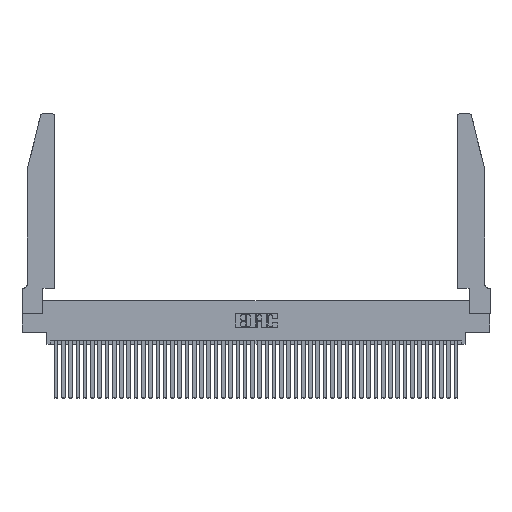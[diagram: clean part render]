
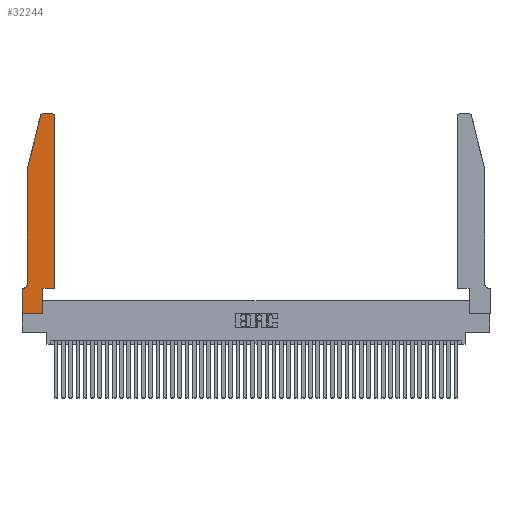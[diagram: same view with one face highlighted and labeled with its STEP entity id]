
A CAD part, top view. The second image highlights one B-rep face of the part: STEP entity #32244.
In plain terms, the highlighted planar face has unit normal (0, 0, 1).
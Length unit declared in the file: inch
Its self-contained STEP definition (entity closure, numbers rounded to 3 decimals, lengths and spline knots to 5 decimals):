
#1064 = EDGE_CURVE ( 'NONE', #2096, #32470, #44818, .T. ) ;
#1934 = DIRECTION ( 'NONE',  ( 0., -1., 0. ) ) ;
#2096 = VERTEX_POINT ( 'NONE', #42912 ) ;
#3128 = ORIENTED_EDGE ( 'NONE', *, *, #29741, .T. ) ;
#4779 = VECTOR ( 'NONE', #26442, 39.37008 ) ;
#6414 = LINE ( 'NONE', #42058, #39681 ) ;
#6590 = VECTOR ( 'NONE', #1934, 39.37008 ) ;
#6786 = CARTESIAN_POINT ( 'NONE',  ( 0.4505, 2.72, 0.37 ) ) ;
#6930 = VECTOR ( 'NONE', #35611, 39.37008 ) ;
#6940 = EDGE_CURVE ( 'NONE', #19842, #30577, #6414, .T. ) ;
#7365 = DIRECTION ( 'NONE',  ( 1., 0., 0. ) ) ;
#8412 = ORIENTED_EDGE ( 'NONE', *, *, #44773, .T. ) ;
#9983 = LINE ( 'NONE', #26506, #6590 ) ;
#10655 = PLANE ( 'NONE',  #27643 ) ;
#12124 = CARTESIAN_POINT ( 'NONE',  ( 0.0755, 0.35, 0.37 ) ) ;
#12376 = CARTESIAN_POINT ( 'NONE',  ( 0.2865, 0.35, 0.37 ) ) ;
#12645 = CARTESIAN_POINT ( 'NONE',  ( 0., 0.35, 0.37 ) ) ;
#13180 = VERTEX_POINT ( 'NONE', #37721 ) ;
#14116 = FACE_OUTER_BOUND ( 'NONE', #36473, .T. ) ;
#14695 = ORIENTED_EDGE ( 'NONE', *, *, #1064, .T. ) ;
#14937 = VECTOR ( 'NONE', #29112, 39.37008 ) ;
#15252 = VERTEX_POINT ( 'NONE', #18741 ) ;
#15470 = LINE ( 'NONE', #26940, #4779 ) ;
#15561 = VECTOR ( 'NONE', #19026, 39.37008 ) ;
#15694 = DIRECTION ( 'NONE',  ( 0., 1., 0. ) ) ;
#15696 = VERTEX_POINT ( 'NONE', #40774 ) ;
#15975 = ORIENTED_EDGE ( 'NONE', *, *, #6940, .T. ) ;
#17004 = ORIENTED_EDGE ( 'NONE', *, *, #36597, .T. ) ;
#17228 = VERTEX_POINT ( 'NONE', #45197 ) ;
#17938 = CARTESIAN_POINT ( 'NONE',  ( 0.4505, 0.35, 0.37 ) ) ;
#18741 = CARTESIAN_POINT ( 'NONE',  ( 0.4505, 0.35, 0.37 ) ) ;
#18858 = CIRCLE ( 'NONE', #31697, 0.03 ) ;
#19026 = DIRECTION ( 'NONE',  ( -0.239, -0.971, 0. ) ) ;
#19027 = DIRECTION ( 'NONE',  ( 0., 0., -1. ) ) ;
#19765 = EDGE_CURVE ( 'NONE', #15252, #45387, #15470, .T. ) ;
#19842 = VERTEX_POINT ( 'NONE', #12645 ) ;
#20671 = LINE ( 'NONE', #29602, #15561 ) ;
#22163 = DIRECTION ( 'NONE',  ( 1., 0., 0. ) ) ;
#23028 = DIRECTION ( 'NONE',  ( 1., 0., 0. ) ) ;
#25004 = DIRECTION ( 'NONE',  ( 1., 0., 0. ) ) ;
#25861 = ORIENTED_EDGE ( 'NONE', *, *, #27218, .T. ) ;
#26118 = ORIENTED_EDGE ( 'NONE', *, *, #19765, .T. ) ;
#26442 = DIRECTION ( 'NONE',  ( 0., 1., 0. ) ) ;
#26506 = CARTESIAN_POINT ( 'NONE',  ( 0.0755, 2., 0.37 ) ) ;
#26940 = CARTESIAN_POINT ( 'NONE',  ( 0.4505, 0.35, 0.37 ) ) ;
#26966 = CARTESIAN_POINT ( 'NONE',  ( 0.284, 2.72, 0.37 ) ) ;
#27079 = EDGE_CURVE ( 'NONE', #32728, #13180, #9983, .T. ) ;
#27218 = EDGE_CURVE ( 'NONE', #17228, #32728, #20671, .T. ) ;
#27497 = CIRCLE ( 'NONE', #28677, 0.03 ) ;
#27643 = AXIS2_PLACEMENT_3D ( 'NONE', #35831, #43468, #7365 ) ;
#27760 = CARTESIAN_POINT ( 'NONE',  ( 0.284, 2.75, 0.37 ) ) ;
#27965 = DIRECTION ( 'NONE',  ( -1., 0., 0. ) ) ;
#28675 = ORIENTED_EDGE ( 'NONE', *, *, #34203, .T. ) ;
#28677 = AXIS2_PLACEMENT_3D ( 'NONE', #29239, #32805, #22163 ) ;
#29112 = DIRECTION ( 'NONE',  ( -1., 0., 0. ) ) ;
#29239 = CARTESIAN_POINT ( 'NONE',  ( 0.4205, 2.72, 0.37 ) ) ;
#29472 = LINE ( 'NONE', #42070, #45372 ) ;
#29602 = CARTESIAN_POINT ( 'NONE',  ( 0.0755, 2., 0.37 ) ) ;
#29741 = EDGE_CURVE ( 'NONE', #32470, #15252, #34557, .T. ) ;
#29920 = CIRCLE ( 'NONE', #37640, 0.07 ) ;
#30577 = VERTEX_POINT ( 'NONE', #39751 ) ;
#31289 = DIRECTION ( 'NONE',  ( 0., -1., 0. ) ) ;
#31697 = AXIS2_PLACEMENT_3D ( 'NONE', #26966, #44699, #23028 ) ;
#32244 = ADVANCED_FACE ( 'NONE', ( #14116 ), #10655, .T. ) ;
#32470 = VERTEX_POINT ( 'NONE', #12376 ) ;
#32543 = CARTESIAN_POINT ( 'NONE',  ( 0., 0., 0.37 ) ) ;
#32728 = VERTEX_POINT ( 'NONE', #35177 ) ;
#32802 = ORIENTED_EDGE ( 'NONE', *, *, #39338, .T. ) ;
#32805 = DIRECTION ( 'NONE',  ( 0., 0., 1. ) ) ;
#34203 = EDGE_CURVE ( 'NONE', #13180, #15696, #29920, .T. ) ;
#34557 = LINE ( 'NONE', #17938, #45388 ) ;
#35177 = CARTESIAN_POINT ( 'NONE',  ( 0.0755, 2., 0.37 ) ) ;
#35377 = VERTEX_POINT ( 'NONE', #36590 ) ;
#35611 = DIRECTION ( 'NONE',  ( 1., 0., 0. ) ) ;
#35831 = CARTESIAN_POINT ( 'NONE',  ( 0., 0.35, 0.37 ) ) ;
#36305 = VECTOR ( 'NONE', #15694, 39.37008 ) ;
#36473 = EDGE_LOOP ( 'NONE', ( #32802, #43476, #25861, #38964, #28675, #36747, #15975, #8412, #14695, #3128, #26118, #17004 ) ) ;
#36590 = CARTESIAN_POINT ( 'NONE',  ( 0.4205, 2.75, 0.37 ) ) ;
#36597 = EDGE_CURVE ( 'NONE', #45387, #35377, #27497, .T. ) ;
#36747 = ORIENTED_EDGE ( 'NONE', *, *, #42180, .T. ) ;
#37640 = AXIS2_PLACEMENT_3D ( 'NONE', #40841, #19027, #41322 ) ;
#37721 = CARTESIAN_POINT ( 'NONE',  ( 0.0755, 0.42, 0.37 ) ) ;
#38042 = EDGE_CURVE ( 'NONE', #44631, #17228, #18858, .T. ) ;
#38964 = ORIENTED_EDGE ( 'NONE', *, *, #27079, .T. ) ;
#39338 = EDGE_CURVE ( 'NONE', #35377, #44631, #29472, .T. ) ;
#39681 = VECTOR ( 'NONE', #31289, 39.37008 ) ;
#39751 = CARTESIAN_POINT ( 'NONE',  ( 0., 0., 0.37 ) ) ;
#40774 = CARTESIAN_POINT ( 'NONE',  ( 0.0055, 0.35, 0.37 ) ) ;
#40841 = CARTESIAN_POINT ( 'NONE',  ( 0.0055, 0.42, 0.37 ) ) ;
#41322 = DIRECTION ( 'NONE',  ( -1., 0., 0. ) ) ;
#42058 = CARTESIAN_POINT ( 'NONE',  ( 0., 0., 0.37 ) ) ;
#42070 = CARTESIAN_POINT ( 'NONE',  ( 0.2605, 2.75, 0.37 ) ) ;
#42180 = EDGE_CURVE ( 'NONE', #15696, #19842, #46605, .T. ) ;
#42912 = CARTESIAN_POINT ( 'NONE',  ( 0.2865, 0., 0.37 ) ) ;
#43468 = DIRECTION ( 'NONE',  ( 0., 0., 1. ) ) ;
#43476 = ORIENTED_EDGE ( 'NONE', *, *, #38042, .T. ) ;
#44631 = VERTEX_POINT ( 'NONE', #27760 ) ;
#44699 = DIRECTION ( 'NONE',  ( 0., 0., 1. ) ) ;
#44712 = LINE ( 'NONE', #32543, #6930 ) ;
#44773 = EDGE_CURVE ( 'NONE', #30577, #2096, #44712, .T. ) ;
#44818 = LINE ( 'NONE', #44943, #36305 ) ;
#44943 = CARTESIAN_POINT ( 'NONE',  ( 0.2865, 0.35, 0.37 ) ) ;
#45197 = CARTESIAN_POINT ( 'NONE',  ( 0.25487, 2.72718, 0.37 ) ) ;
#45372 = VECTOR ( 'NONE', #27965, 39.37008 ) ;
#45387 = VERTEX_POINT ( 'NONE', #6786 ) ;
#45388 = VECTOR ( 'NONE', #25004, 39.37008 ) ;
#46605 = LINE ( 'NONE', #12124, #14937 ) ;
